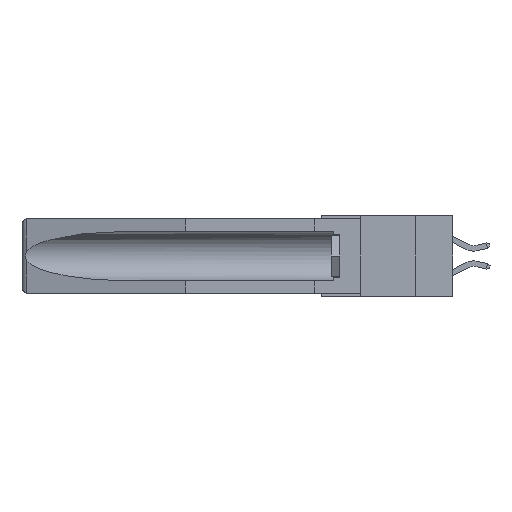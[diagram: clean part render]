
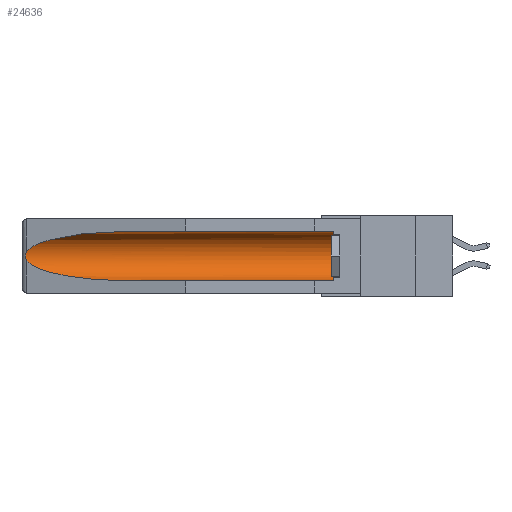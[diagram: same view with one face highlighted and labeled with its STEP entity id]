
A CAD part, left-side view. The second image highlights one B-rep face of the part: STEP entity #24636.
In plain terms, the highlighted cylindrical face has radius 2.857 mm (diameter 5.715 mm), a partial arc.
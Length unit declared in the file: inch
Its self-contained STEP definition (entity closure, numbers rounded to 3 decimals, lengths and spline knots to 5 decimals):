
#1477 = CARTESIAN_POINT ( 'NONE',  ( 0.155, -0.30754, -0.284 ) ) ;
#2014 = CARTESIAN_POINT ( 'NONE',  ( 0.155, 0.126, -0.059 ) ) ;
#3128 = EDGE_CURVE ( 'NONE', #19912, #9525, #25135, .T. ) ;
#3597 = VECTOR ( 'NONE', #13332, 39.37008 ) ;
#3862 = CARTESIAN_POINT ( 'NONE',  ( 0.26537, 1.52718, -0.14972 ) ) ;
#3981 = ORIENTED_EDGE ( 'NONE', *, *, #4850, .T. ) ;
#4151 = DIRECTION ( 'NONE',  ( 0., 0., 1. ) ) ;
#4584 = CARTESIAN_POINT ( 'NONE',  ( 0.21114, 1.30732, -0.059 ) ) ;
#4850 = EDGE_CURVE ( 'NONE', #6780, #24338, #23760, .T. ) ;
#5243 = ORIENTED_EDGE ( 'NONE', *, *, #3128, .T. ) ;
#5251 = ORIENTED_EDGE ( 'NONE', *, *, #7932, .T. ) ;
#5895 = CARTESIAN_POINT ( 'NONE',  ( 0.155, 1.07973, -0.059 ) ) ;
#6780 = VERTEX_POINT ( 'NONE', #5895 ) ;
#7663 = CARTESIAN_POINT ( 'NONE',  ( 0.26655, 1.53094, -0.18657 ) ) ;
#7932 = EDGE_CURVE ( 'NONE', #21972, #8661, #8046, .T. ) ;
#8014 = CARTESIAN_POINT ( 'NONE',  ( 0.25451, 1.48313, -0.24835 ) ) ;
#8046 =( BOUNDED_CURVE ( )  B_SPLINE_CURVE ( 3, ( #18220, #8014, #23858, #17954 ),
 .UNSPECIFIED., .F., .F. ) 
 B_SPLINE_CURVE_WITH_KNOTS ( ( 4, 4 ),
 ( 0.1948, 1.5708 ),
 .UNSPECIFIED. ) 
 CURVE ( )  GEOMETRIC_REPRESENTATION_ITEM ( )  RATIONAL_B_SPLINE_CURVE ( ( 1., 0.848, 0.848, 1. ) ) 
 REPRESENTATION_ITEM ( '' )  );
#8211 = EDGE_LOOP ( 'NONE', ( #3981, #13059, #5251, #15515, #5243, #21113 ) ) ;
#8661 = VERTEX_POINT ( 'NONE', #9246 ) ;
#9246 = CARTESIAN_POINT ( 'NONE',  ( 0.155, 1.07973, -0.284 ) ) ;
#9525 = VERTEX_POINT ( 'NONE', #2014 ) ;
#9556 = CARTESIAN_POINT ( 'NONE',  ( 0.26537, 1.52718, -0.19328 ) ) ;
#9876 = EDGE_CURVE ( 'NONE', #9525, #6780, #11497, .T. ) ;
#10755 = DIRECTION ( 'NONE',  ( 0., 0., 1. ) ) ;
#11264 = DIRECTION ( 'NONE',  ( 0., 1., 0. ) ) ;
#11497 = LINE ( 'NONE', #16811, #14893 ) ;
#11873 = EDGE_CURVE ( 'NONE', #24338, #21972, #16934, .T. ) ;
#12691 = CARTESIAN_POINT ( 'NONE',  ( 0.155, 1.07973, -0.059 ) ) ;
#13059 = ORIENTED_EDGE ( 'NONE', *, *, #11873, .T. ) ;
#13332 = DIRECTION ( 'NONE',  ( 0., 1., 0. ) ) ;
#13992 = DIRECTION ( 'NONE',  ( 0., -1., 0. ) ) ;
#14022 = FACE_OUTER_BOUND ( 'NONE', #8211, .T. ) ;
#14687 = CARTESIAN_POINT ( 'NONE',  ( 0.25451, 1.48313, -0.09465 ) ) ;
#14893 = VECTOR ( 'NONE', #11264, 39.37008 ) ;
#15515 = ORIENTED_EDGE ( 'NONE', *, *, #23485, .F. ) ;
#15803 = CARTESIAN_POINT ( 'NONE',  ( 0.155, 0.126, -0.1715 ) ) ;
#16245 = LINE ( 'NONE', #1477, #3597 ) ;
#16677 = CARTESIAN_POINT ( 'NONE',  ( 0.26537, 1.52718, -0.14972 ) ) ;
#16811 = CARTESIAN_POINT ( 'NONE',  ( 0.155, -0.30754, -0.059 ) ) ;
#16934 = B_SPLINE_CURVE_WITH_KNOTS ( 'NONE', 3,
 ( #3862, #17702, #25684, #17621, #21679, #19620, #17372, #7663, #19534, #9556 ),
 .UNSPECIFIED., .F., .F.,
 ( 4, 2, 2, 2, 4 ),
 ( 0., 0.00029, 0.00058, 0.00087, 0.00117 ),
 .UNSPECIFIED. ) ;
#17372 = CARTESIAN_POINT ( 'NONE',  ( 0.2673, 1.53269, -0.17917 ) ) ;
#17621 = CARTESIAN_POINT ( 'NONE',  ( 0.2673, 1.5327, -0.16383 ) ) ;
#17702 = CARTESIAN_POINT ( 'NONE',  ( 0.26597, 1.52961, -0.15275 ) ) ;
#17954 = CARTESIAN_POINT ( 'NONE',  ( 0.155, 1.07973, -0.284 ) ) ;
#18054 = CYLINDRICAL_SURFACE ( 'NONE', #25205, 0.1125 ) ;
#18220 = CARTESIAN_POINT ( 'NONE',  ( 0.26537, 1.52718, -0.19328 ) ) ;
#18240 = AXIS2_PLACEMENT_3D ( 'NONE', #15803, #13992, #4151 ) ;
#19534 = CARTESIAN_POINT ( 'NONE',  ( 0.26597, 1.5296, -0.19026 ) ) ;
#19620 = CARTESIAN_POINT ( 'NONE',  ( 0.2675, 1.53308, -0.17534 ) ) ;
#19878 = CARTESIAN_POINT ( 'NONE',  ( 0.26537, 1.52718, -0.14972 ) ) ;
#19912 = VERTEX_POINT ( 'NONE', #21074 ) ;
#20542 = CARTESIAN_POINT ( 'NONE',  ( 0.155, -0.30754, -0.1715 ) ) ;
#21074 = CARTESIAN_POINT ( 'NONE',  ( 0.155, 0.126, -0.284 ) ) ;
#21113 = ORIENTED_EDGE ( 'NONE', *, *, #9876, .T. ) ;
#21679 = CARTESIAN_POINT ( 'NONE',  ( 0.2675, 1.53308, -0.16763 ) ) ;
#21972 = VERTEX_POINT ( 'NONE', #22845 ) ;
#22644 = DIRECTION ( 'NONE',  ( 0., 1., 0. ) ) ;
#22845 = CARTESIAN_POINT ( 'NONE',  ( 0.26537, 1.52718, -0.19328 ) ) ;
#23485 = EDGE_CURVE ( 'NONE', #19912, #8661, #16245, .T. ) ;
#23760 =( BOUNDED_CURVE ( )  B_SPLINE_CURVE ( 3, ( #12691, #4584, #14687, #16677 ),
 .UNSPECIFIED., .F., .F. ) 
 B_SPLINE_CURVE_WITH_KNOTS ( ( 4, 4 ),
 ( 4.71239, 6.08839 ),
 .UNSPECIFIED. ) 
 CURVE ( )  GEOMETRIC_REPRESENTATION_ITEM ( )  RATIONAL_B_SPLINE_CURVE ( ( 1., 0.848, 0.848, 1. ) ) 
 REPRESENTATION_ITEM ( '' )  );
#23858 = CARTESIAN_POINT ( 'NONE',  ( 0.21114, 1.30732, -0.284 ) ) ;
#24338 = VERTEX_POINT ( 'NONE', #19878 ) ;
#24636 = ADVANCED_FACE ( 'NONE', ( #14022 ), #18054, .F. ) ;
#25135 = CIRCLE ( 'NONE', #18240, 0.1125 ) ;
#25205 = AXIS2_PLACEMENT_3D ( 'NONE', #20542, #22644, #10755 ) ;
#25684 = CARTESIAN_POINT ( 'NONE',  ( 0.26654, 1.53092, -0.15636 ) ) ;
